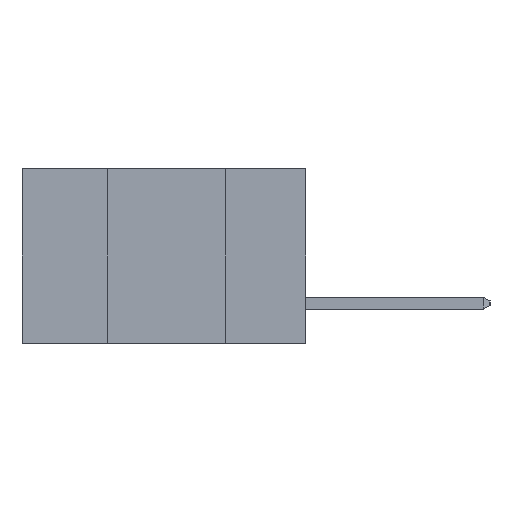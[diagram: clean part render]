
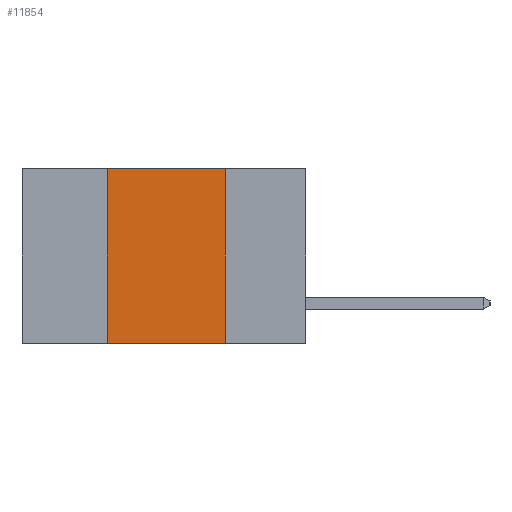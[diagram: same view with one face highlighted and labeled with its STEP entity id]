
A CAD part, left-side view. The second image highlights one B-rep face of the part: STEP entity #11854.
In plain terms, the highlighted planar face has unit normal (-1, 0, 0).
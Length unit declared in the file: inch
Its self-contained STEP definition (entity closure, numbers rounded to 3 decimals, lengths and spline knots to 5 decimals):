
#507 = EDGE_LOOP ( 'NONE', ( #19988, #11278, #874, #13237 ) ) ;
#874 = ORIENTED_EDGE ( 'NONE', *, *, #17915, .F. ) ;
#1925 = EDGE_CURVE ( 'NONE', #14094, #8222, #21521, .T. ) ;
#2770 = CARTESIAN_POINT ( 'NONE',  ( 0., 0.17, 0. ) ) ;
#2796 = DIRECTION ( 'NONE',  ( 0., 0., -1. ) ) ;
#3352 = LINE ( 'NONE', #17910, #8225 ) ;
#3621 = DIRECTION ( 'NONE',  ( 0., 0., 1. ) ) ;
#4900 = LINE ( 'NONE', #9830, #15267 ) ;
#4955 = CARTESIAN_POINT ( 'NONE',  ( 0., 0.6, 0. ) ) ;
#6076 = EDGE_CURVE ( 'NONE', #20594, #14094, #3352, .T. ) ;
#6998 = DIRECTION ( 'NONE',  ( 0., 0., -1. ) ) ;
#7209 = CARTESIAN_POINT ( 'NONE',  ( 0., 0.42, -0.37 ) ) ;
#8222 = VERTEX_POINT ( 'NONE', #12188 ) ;
#8225 = VECTOR ( 'NONE', #12521, 39.37008 ) ;
#9830 = CARTESIAN_POINT ( 'NONE',  ( 0., 0.6, -0.37 ) ) ;
#9974 = VECTOR ( 'NONE', #3621, 39.37008 ) ;
#11278 = ORIENTED_EDGE ( 'NONE', *, *, #6076, .F. ) ;
#11854 = ADVANCED_FACE ( 'NONE', ( #12491 ), #23246, .F. ) ;
#11933 = DIRECTION ( 'NONE',  ( 0., -1., 0. ) ) ;
#12188 = CARTESIAN_POINT ( 'NONE',  ( 0., 0.17, -0.37 ) ) ;
#12491 = FACE_OUTER_BOUND ( 'NONE', #507, .T. ) ;
#12521 = DIRECTION ( 'NONE',  ( 0., -1., 0. ) ) ;
#13237 = ORIENTED_EDGE ( 'NONE', *, *, #20840, .T. ) ;
#14094 = VERTEX_POINT ( 'NONE', #14330 ) ;
#14330 = CARTESIAN_POINT ( 'NONE',  ( 0., 0.17, 0. ) ) ;
#15267 = VECTOR ( 'NONE', #11933, 39.37008 ) ;
#15439 = LINE ( 'NONE', #25876, #9974 ) ;
#17910 = CARTESIAN_POINT ( 'NONE',  ( 0., 0.6, 0. ) ) ;
#17915 = EDGE_CURVE ( 'NONE', #18350, #20594, #15439, .T. ) ;
#18350 = VERTEX_POINT ( 'NONE', #7209 ) ;
#19351 = DIRECTION ( 'NONE',  ( 1., 0., 0. ) ) ;
#19988 = ORIENTED_EDGE ( 'NONE', *, *, #1925, .F. ) ;
#20594 = VERTEX_POINT ( 'NONE', #23125 ) ;
#20840 = EDGE_CURVE ( 'NONE', #18350, #8222, #4900, .T. ) ;
#20903 = VECTOR ( 'NONE', #2796, 39.37008 ) ;
#21521 = LINE ( 'NONE', #2770, #20903 ) ;
#23125 = CARTESIAN_POINT ( 'NONE',  ( 0., 0.42, 0. ) ) ;
#23246 = PLANE ( 'NONE',  #24766 ) ;
#24766 = AXIS2_PLACEMENT_3D ( 'NONE', #4955, #19351, #6998 ) ;
#25876 = CARTESIAN_POINT ( 'NONE',  ( 0., 0.42, 0. ) ) ;
